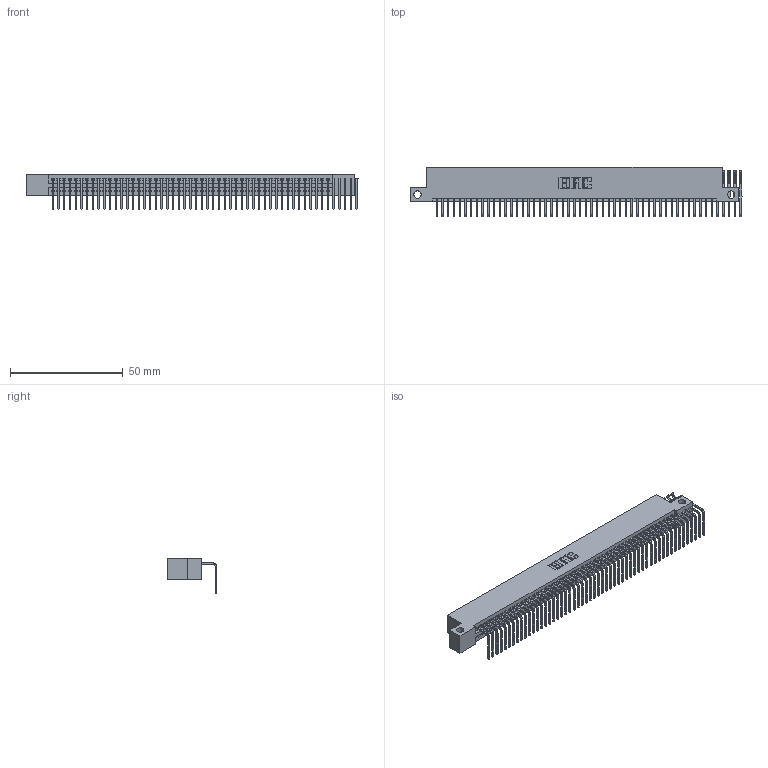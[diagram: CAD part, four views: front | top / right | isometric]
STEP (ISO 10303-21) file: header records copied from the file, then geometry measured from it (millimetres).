
FILE_DESCRIPTION (( 'STEP AP203' ), '1' );
FILE_NAME ('345-054-558-112.STEP', '2019-10-10T19:11:58', ( '' ), ( '' ), 'SwSTEP 2.0', 'SolidWorks 2016', '' );
FILE_SCHEMA (( 'CONFIG_CONTROL_DESIGN' ));
Length unit declared in the file: inch
Products named in the file (3): 345 Part_Flush Mounting Lugs - Side Mount; 345-292-001_558 Tail - 2; 345-054-558-112
Assembly tree (55 placements, depth 2):
  345-054-558-112
    345 Part_Flush Mounting Lugs - Side Mount
    345-292-001_558 Tail - 2  x54
Bounding box: 147.13 x 21.83 x 15.37 mm (x, y, z)
Volume: 14043 mm3; surface area: 19976.3 mm2
Topology: 55 solids, 55 shells, 3286 faces, 9899 edges, 6526 vertices
Faces by surface type: plane 2278, cylinder 1008
Entity records: 36183 total; most frequent: CARTESIAN_POINT 6252, ORIENTED_EDGE 6230, DIRECTION 5455, EDGE_CURVE 3115, VECTOR 2787, LINE 2787, VERTEX_POINT 2074, AXIS2_PLACEMENT_3D 1334
